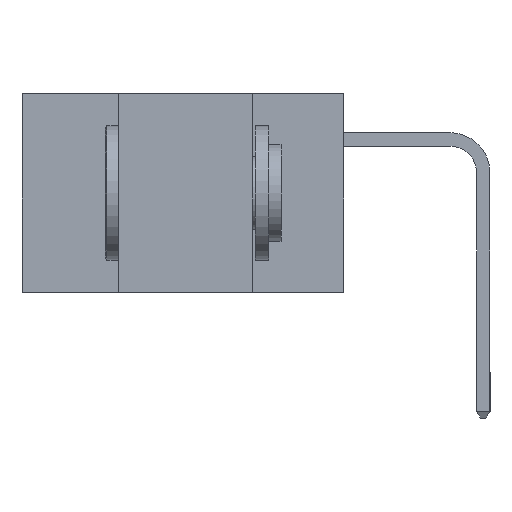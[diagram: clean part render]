
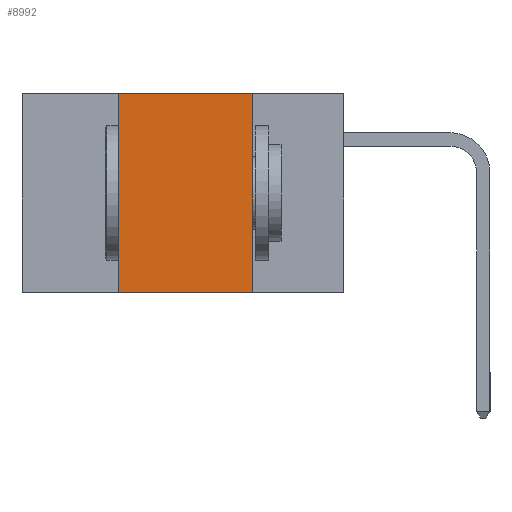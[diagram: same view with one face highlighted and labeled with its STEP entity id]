
A CAD part, left-side view. The second image highlights one B-rep face of the part: STEP entity #8992.
In plain terms, the highlighted planar face has unit normal (-1, 0, 0).
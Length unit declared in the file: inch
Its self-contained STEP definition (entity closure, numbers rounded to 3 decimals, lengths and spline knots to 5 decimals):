
#52 = DIRECTION ( 'NONE',  ( 0., 0., -1. ) ) ;
#288 = DIRECTION ( 'NONE',  ( 0., 0., 1. ) ) ;
#509 = ORIENTED_EDGE ( 'NONE', *, *, #8232, .T. ) ;
#1801 = VECTOR ( 'NONE', #288, 39.37008 ) ;
#1809 = CARTESIAN_POINT ( 'NONE',  ( 0., 0.42, 0. ) ) ;
#2000 = CARTESIAN_POINT ( 'NONE',  ( 0., 0.6, 0. ) ) ;
#2115 = VERTEX_POINT ( 'NONE', #14408 ) ;
#3030 = ORIENTED_EDGE ( 'NONE', *, *, #19158, .F. ) ;
#3389 = DIRECTION ( 'NONE',  ( 0., 0., -1. ) ) ;
#3407 = DIRECTION ( 'NONE',  ( 0., -1., 0. ) ) ;
#4113 = VERTEX_POINT ( 'NONE', #5309 ) ;
#4134 = PLANE ( 'NONE',  #19033 ) ;
#4286 = VECTOR ( 'NONE', #15416, 39.37008 ) ;
#4386 = LINE ( 'NONE', #18294, #9439 ) ;
#4886 = CARTESIAN_POINT ( 'NONE',  ( 0., 0.6, 0. ) ) ;
#5309 = CARTESIAN_POINT ( 'NONE',  ( 0., 0.17, -0.37 ) ) ;
#5582 = CARTESIAN_POINT ( 'NONE',  ( 0., 0.42, -0.37 ) ) ;
#7503 = ORIENTED_EDGE ( 'NONE', *, *, #9121, .F. ) ;
#7610 = FACE_OUTER_BOUND ( 'NONE', #19005, .T. ) ;
#8232 = EDGE_CURVE ( 'NONE', #17971, #4113, #11982, .T. ) ;
#8992 = ADVANCED_FACE ( 'NONE', ( #7610 ), #4134, .F. ) ;
#9121 = EDGE_CURVE ( 'NONE', #13710, #2115, #10995, .T. ) ;
#9439 = VECTOR ( 'NONE', #52, 39.37008 ) ;
#10979 = DIRECTION ( 'NONE',  ( 1., 0., 0. ) ) ;
#10995 = LINE ( 'NONE', #2000, #19382 ) ;
#11982 = LINE ( 'NONE', #15321, #4286 ) ;
#12414 = LINE ( 'NONE', #18541, #1801 ) ;
#12983 = ORIENTED_EDGE ( 'NONE', *, *, #14033, .F. ) ;
#13710 = VERTEX_POINT ( 'NONE', #1809 ) ;
#14033 = EDGE_CURVE ( 'NONE', #2115, #4113, #4386, .T. ) ;
#14408 = CARTESIAN_POINT ( 'NONE',  ( 0., 0.17, 0. ) ) ;
#15321 = CARTESIAN_POINT ( 'NONE',  ( 0., 0.6, -0.37 ) ) ;
#15416 = DIRECTION ( 'NONE',  ( 0., -1., 0. ) ) ;
#17971 = VERTEX_POINT ( 'NONE', #5582 ) ;
#18294 = CARTESIAN_POINT ( 'NONE',  ( 0., 0.17, -0.37 ) ) ;
#18541 = CARTESIAN_POINT ( 'NONE',  ( 0., 0.42, -0.37 ) ) ;
#19005 = EDGE_LOOP ( 'NONE', ( #12983, #7503, #3030, #509 ) ) ;
#19033 = AXIS2_PLACEMENT_3D ( 'NONE', #4886, #10979, #3389 ) ;
#19158 = EDGE_CURVE ( 'NONE', #17971, #13710, #12414, .T. ) ;
#19382 = VECTOR ( 'NONE', #3407, 39.37008 ) ;
